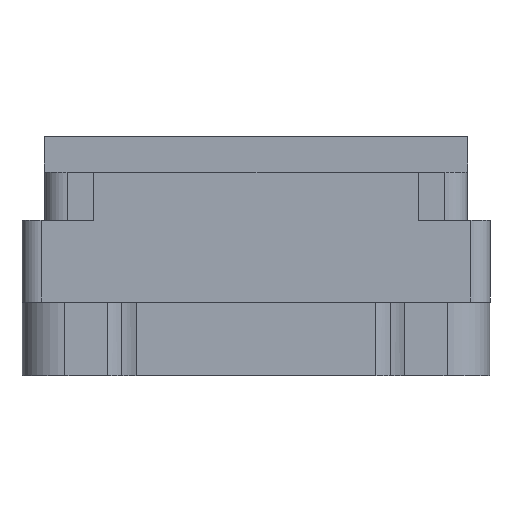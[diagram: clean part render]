
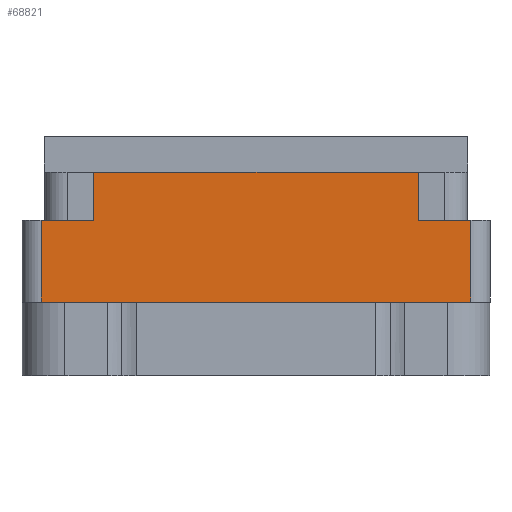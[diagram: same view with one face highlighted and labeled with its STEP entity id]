
A CAD part, left-side view. The second image highlights one B-rep face of the part: STEP entity #68821.
In plain terms, the highlighted planar face has unit normal (-1, 0, 0).
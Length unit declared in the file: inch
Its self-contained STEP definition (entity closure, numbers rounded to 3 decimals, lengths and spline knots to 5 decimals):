
#760 = ORIENTED_EDGE ( 'NONE', *, *, #18201, .F. ) ;
#1260 = DIRECTION ( 'NONE',  ( 0., -1., 0. ) ) ;
#1720 = LINE ( 'NONE', #78446, #40583 ) ;
#1749 = EDGE_CURVE ( 'NONE', #76112, #69226, #13037, .T. ) ;
#1781 = CARTESIAN_POINT ( 'NONE',  ( -1.375, 0.5285, -0.274 ) ) ;
#2514 = ORIENTED_EDGE ( 'NONE', *, *, #12896, .F. ) ;
#2655 = VECTOR ( 'NONE', #44221, 39.37008 ) ;
#3767 = EDGE_CURVE ( 'NONE', #75798, #51912, #65123, .T. ) ;
#5338 = DIRECTION ( 'NONE',  ( 0., -1., 0. ) ) ;
#6582 = CARTESIAN_POINT ( 'NONE',  ( -1.375, 0., -0.54 ) ) ;
#12012 = LINE ( 'NONE', #45159, #19921 ) ;
#12896 = EDGE_CURVE ( 'NONE', #76112, #45011, #49928, .T. ) ;
#13037 = LINE ( 'NONE', #27857, #47963 ) ;
#16405 = ORIENTED_EDGE ( 'NONE', *, *, #3767, .T. ) ;
#17723 = EDGE_CURVE ( 'NONE', #24516, #49322, #12012, .T. ) ;
#18201 = EDGE_CURVE ( 'NONE', #49322, #69226, #37297, .T. ) ;
#18540 = VECTOR ( 'NONE', #1260, 39.37008 ) ;
#19921 = VECTOR ( 'NONE', #63348, 39.37008 ) ;
#20060 = ORIENTED_EDGE ( 'NONE', *, *, #74709, .F. ) ;
#20843 = VERTEX_POINT ( 'NONE', #57172 ) ;
#21791 = EDGE_CURVE ( 'NONE', #51912, #20843, #35683, .T. ) ;
#22770 = DIRECTION ( 'NONE',  ( 0., 0., 1. ) ) ;
#23745 = DIRECTION ( 'NONE',  ( 0., 0., 1. ) ) ;
#24516 = VERTEX_POINT ( 'NONE', #1781 ) ;
#26959 = CARTESIAN_POINT ( 'NONE',  ( -1.375, -0.5285, -0.117 ) ) ;
#27857 = CARTESIAN_POINT ( 'NONE',  ( -1.375, -0.5285, -0.274 ) ) ;
#29717 = EDGE_CURVE ( 'NONE', #20843, #45011, #1720, .T. ) ;
#31378 = AXIS2_PLACEMENT_3D ( 'NONE', #78283, #38938, #22770 ) ;
#35683 = LINE ( 'NONE', #6582, #2655 ) ;
#36901 = EDGE_LOOP ( 'NONE', ( #20060, #16405, #50717, #41116, #2514, #39168, #760, #69297 ) ) ;
#37297 = LINE ( 'NONE', #47870, #55736 ) ;
#38938 = DIRECTION ( 'NONE',  ( -1., 0., 0. ) ) ;
#39130 = FACE_OUTER_BOUND ( 'NONE', #36901, .T. ) ;
#39168 = ORIENTED_EDGE ( 'NONE', *, *, #1749, .T. ) ;
#40583 = VECTOR ( 'NONE', #23745, 39.37008 ) ;
#41116 = ORIENTED_EDGE ( 'NONE', *, *, #29717, .T. ) ;
#44221 = DIRECTION ( 'NONE',  ( 0., -1., 0. ) ) ;
#45011 = VERTEX_POINT ( 'NONE', #68379 ) ;
#45159 = CARTESIAN_POINT ( 'NONE',  ( -1.375, 0.5285, -0.274 ) ) ;
#47870 = CARTESIAN_POINT ( 'NONE',  ( -1.375, 0.7625, -0.117 ) ) ;
#47963 = VECTOR ( 'NONE', #65228, 39.37008 ) ;
#49322 = VERTEX_POINT ( 'NONE', #58233 ) ;
#49928 = LINE ( 'NONE', #65638, #57756 ) ;
#50717 = ORIENTED_EDGE ( 'NONE', *, *, #21791, .T. ) ;
#51912 = VERTEX_POINT ( 'NONE', #75222 ) ;
#52480 = VECTOR ( 'NONE', #53127, 39.37008 ) ;
#53127 = DIRECTION ( 'NONE',  ( 0., 0., -1. ) ) ;
#55736 = VECTOR ( 'NONE', #5338, 39.37008 ) ;
#57172 = CARTESIAN_POINT ( 'NONE',  ( -1.375, -0.7005, -0.54 ) ) ;
#57756 = VECTOR ( 'NONE', #71586, 39.37008 ) ;
#58233 = CARTESIAN_POINT ( 'NONE',  ( -1.375, 0.5285, -0.117 ) ) ;
#59114 = CARTESIAN_POINT ( 'NONE',  ( -1.375, 0.7005, -0.78 ) ) ;
#63348 = DIRECTION ( 'NONE',  ( 0., 0., 1. ) ) ;
#65058 = CARTESIAN_POINT ( 'NONE',  ( -1.375, -0.5285, -0.274 ) ) ;
#65123 = LINE ( 'NONE', #59114, #52480 ) ;
#65228 = DIRECTION ( 'NONE',  ( 0., 0., 1. ) ) ;
#65638 = CARTESIAN_POINT ( 'NONE',  ( -1.375, 0., -0.274 ) ) ;
#68379 = CARTESIAN_POINT ( 'NONE',  ( -1.375, -0.7005, -0.274 ) ) ;
#68539 = CARTESIAN_POINT ( 'NONE',  ( -1.375, 0., -0.274 ) ) ;
#68821 = ADVANCED_FACE ( 'NONE', ( #39130 ), #77473, .T. ) ;
#69226 = VERTEX_POINT ( 'NONE', #26959 ) ;
#69297 = ORIENTED_EDGE ( 'NONE', *, *, #17723, .F. ) ;
#71586 = DIRECTION ( 'NONE',  ( 0., -1., 0. ) ) ;
#74660 = LINE ( 'NONE', #68539, #18540 ) ;
#74709 = EDGE_CURVE ( 'NONE', #75798, #24516, #74660, .T. ) ;
#75111 = CARTESIAN_POINT ( 'NONE',  ( -1.375, 0.7005, -0.274 ) ) ;
#75222 = CARTESIAN_POINT ( 'NONE',  ( -1.375, 0.7005, -0.54 ) ) ;
#75798 = VERTEX_POINT ( 'NONE', #75111 ) ;
#76112 = VERTEX_POINT ( 'NONE', #65058 ) ;
#77473 = PLANE ( 'NONE',  #31378 ) ;
#78283 = CARTESIAN_POINT ( 'NONE',  ( -1.375, -0.7625, -0.78 ) ) ;
#78446 = CARTESIAN_POINT ( 'NONE',  ( -1.375, -0.7005, -0.78 ) ) ;
